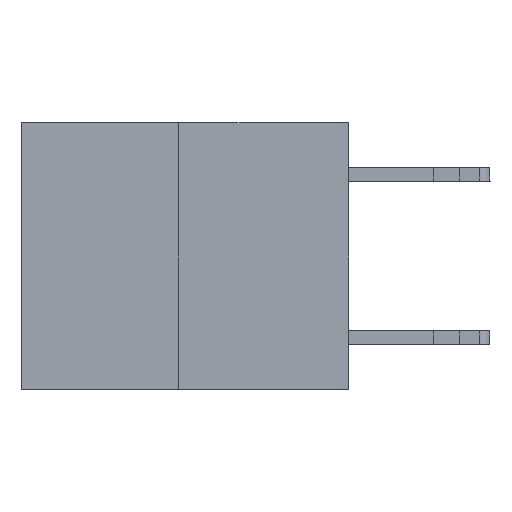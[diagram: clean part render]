
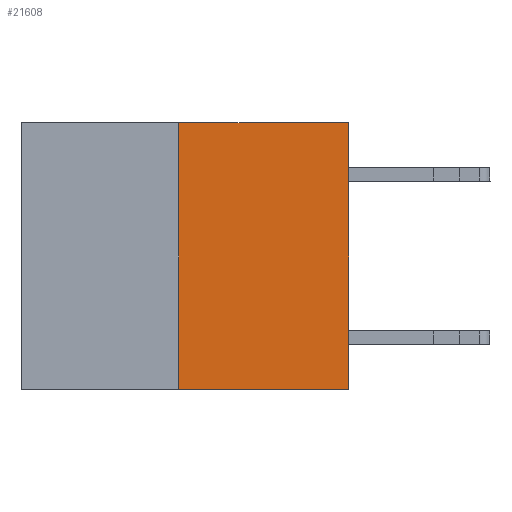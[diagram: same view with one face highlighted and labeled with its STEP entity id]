
A CAD part, left-side view. The second image highlights one B-rep face of the part: STEP entity #21608.
In plain terms, the highlighted planar face has unit normal (-1, 0, 0).
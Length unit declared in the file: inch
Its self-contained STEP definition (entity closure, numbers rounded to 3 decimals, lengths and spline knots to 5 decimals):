
#518 = CARTESIAN_POINT ( 'NONE',  ( 0., 0., -0.49 ) ) ;
#574 = VECTOR ( 'NONE', #3071, 39.37008 ) ;
#3071 = DIRECTION ( 'NONE',  ( 0., -1., 0. ) ) ;
#4520 = VERTEX_POINT ( 'NONE', #4842 ) ;
#4842 = CARTESIAN_POINT ( 'NONE',  ( 0., 0.312, 0. ) ) ;
#5138 = LINE ( 'NONE', #12211, #21726 ) ;
#5270 = EDGE_CURVE ( 'NONE', #6872, #17932, #10359, .T. ) ;
#5360 = EDGE_CURVE ( 'NONE', #4520, #9482, #19600, .T. ) ;
#5517 = FACE_OUTER_BOUND ( 'NONE', #6331, .T. ) ;
#6331 = EDGE_LOOP ( 'NONE', ( #14557, #12177, #12759, #21388 ) ) ;
#6416 = CARTESIAN_POINT ( 'NONE',  ( 0., 0.312, -0.49 ) ) ;
#6872 = VERTEX_POINT ( 'NONE', #6416 ) ;
#9482 = VERTEX_POINT ( 'NONE', #13166 ) ;
#10359 = LINE ( 'NONE', #13539, #574 ) ;
#11902 = DIRECTION ( 'NONE',  ( 0., 0., 1. ) ) ;
#12177 = ORIENTED_EDGE ( 'NONE', *, *, #5270, .T. ) ;
#12211 = CARTESIAN_POINT ( 'NONE',  ( 0., 0.312, -0.49 ) ) ;
#12404 = VECTOR ( 'NONE', #11902, 39.37008 ) ;
#12759 = ORIENTED_EDGE ( 'NONE', *, *, #15450, .T. ) ;
#13166 = CARTESIAN_POINT ( 'NONE',  ( 0., 0., 0. ) ) ;
#13539 = CARTESIAN_POINT ( 'NONE',  ( 0., 0.6, -0.49 ) ) ;
#13755 = DIRECTION ( 'NONE',  ( 0., 0., 1. ) ) ;
#14557 = ORIENTED_EDGE ( 'NONE', *, *, #18231, .F. ) ;
#15134 = LINE ( 'NONE', #22369, #12404 ) ;
#15450 = EDGE_CURVE ( 'NONE', #17932, #9482, #15134, .T. ) ;
#16939 = CARTESIAN_POINT ( 'NONE',  ( 0., 0.6, 0. ) ) ;
#17015 = DIRECTION ( 'NONE',  ( 1., 0., 0. ) ) ;
#17777 = CARTESIAN_POINT ( 'NONE',  ( 0., 0.6, 0. ) ) ;
#17932 = VERTEX_POINT ( 'NONE', #518 ) ;
#17958 = VECTOR ( 'NONE', #18396, 39.37008 ) ;
#18231 = EDGE_CURVE ( 'NONE', #6872, #4520, #5138, .T. ) ;
#18396 = DIRECTION ( 'NONE',  ( 0., -1., 0. ) ) ;
#18821 = PLANE ( 'NONE',  #20941 ) ;
#19600 = LINE ( 'NONE', #17777, #17958 ) ;
#20941 = AXIS2_PLACEMENT_3D ( 'NONE', #16939, #17015, #22164 ) ;
#21388 = ORIENTED_EDGE ( 'NONE', *, *, #5360, .F. ) ;
#21608 = ADVANCED_FACE ( 'NONE', ( #5517 ), #18821, .F. ) ;
#21726 = VECTOR ( 'NONE', #13755, 39.37008 ) ;
#22164 = DIRECTION ( 'NONE',  ( 0., 0., -1. ) ) ;
#22369 = CARTESIAN_POINT ( 'NONE',  ( 0., 0., 0. ) ) ;
